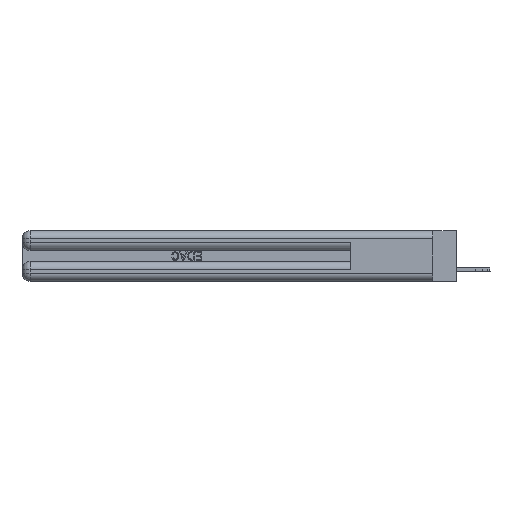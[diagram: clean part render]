
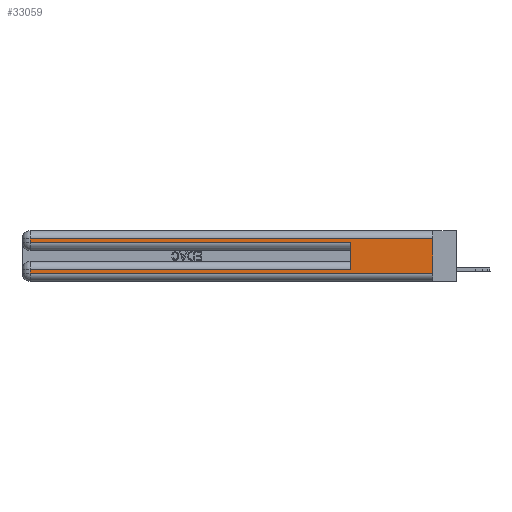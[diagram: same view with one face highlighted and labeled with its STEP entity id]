
A CAD part, left-side view. The second image highlights one B-rep face of the part: STEP entity #33059.
In plain terms, the highlighted planar face has unit normal (-1, 0, 0).
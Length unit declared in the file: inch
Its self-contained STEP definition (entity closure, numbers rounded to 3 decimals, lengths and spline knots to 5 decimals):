
#1173 = EDGE_CURVE ( 'NONE', #10407, #36564, #16976, .T. ) ;
#1502 = VECTOR ( 'NONE', #7105, 39.37008 ) ;
#1995 = ORIENTED_EDGE ( 'NONE', *, *, #1173, .T. ) ;
#2170 = DIRECTION ( 'NONE',  ( 0., -1., 0. ) ) ;
#2304 = VERTEX_POINT ( 'NONE', #34217 ) ;
#2325 = CARTESIAN_POINT ( 'NONE',  ( 0., 2.94, 0.37 ) ) ;
#3157 = DIRECTION ( 'NONE',  ( 0., 0., 1. ) ) ;
#3368 = LINE ( 'NONE', #25558, #22544 ) ;
#4999 = DIRECTION ( 'NONE',  ( 0., 1., 0. ) ) ;
#5261 = CARTESIAN_POINT ( 'NONE',  ( 0., 0., 0.085 ) ) ;
#6459 = ORIENTED_EDGE ( 'NONE', *, *, #23869, .T. ) ;
#6696 = VECTOR ( 'NONE', #2170, 39.37008 ) ;
#7105 = DIRECTION ( 'NONE',  ( 0., -1., 0. ) ) ;
#8098 = VECTOR ( 'NONE', #4999, 39.37008 ) ;
#8385 = CARTESIAN_POINT ( 'NONE',  ( 0., 2.94, 0.06 ) ) ;
#8729 = DIRECTION ( 'NONE',  ( 0., 0., -1. ) ) ;
#8767 = AXIS2_PLACEMENT_3D ( 'NONE', #23512, #29400, #26526 ) ;
#8799 = CARTESIAN_POINT ( 'NONE',  ( 0., 0., 0.06 ) ) ;
#9273 = LINE ( 'NONE', #2325, #12590 ) ;
#9824 = EDGE_CURVE ( 'NONE', #2304, #36564, #22189, .T. ) ;
#10045 = FACE_OUTER_BOUND ( 'NONE', #35761, .T. ) ;
#10250 = VECTOR ( 'NONE', #26584, 39.37008 ) ;
#10407 = VERTEX_POINT ( 'NONE', #11506 ) ;
#11506 = CARTESIAN_POINT ( 'NONE',  ( 0., 2.94, 0.285 ) ) ;
#11939 = ORIENTED_EDGE ( 'NONE', *, *, #13245, .F. ) ;
#12012 = ORIENTED_EDGE ( 'NONE', *, *, #12618, .T. ) ;
#12515 = VERTEX_POINT ( 'NONE', #8385 ) ;
#12590 = VECTOR ( 'NONE', #23504, 39.37008 ) ;
#12618 = EDGE_CURVE ( 'NONE', #2304, #25519, #18220, .T. ) ;
#13245 = EDGE_CURVE ( 'NONE', #35081, #17777, #35471, .T. ) ;
#13804 = DIRECTION ( 'NONE',  ( 0., 0., -1. ) ) ;
#13826 = ORIENTED_EDGE ( 'NONE', *, *, #18901, .T. ) ;
#15466 = CARTESIAN_POINT ( 'NONE',  ( 0., 0.6, 0.285 ) ) ;
#15667 = VECTOR ( 'NONE', #3157, 39.37008 ) ;
#15767 = CARTESIAN_POINT ( 'NONE',  ( 0., 2.94, 0.085 ) ) ;
#16155 = CARTESIAN_POINT ( 'NONE',  ( 0., 0., 0.285 ) ) ;
#16976 = LINE ( 'NONE', #16155, #1502 ) ;
#17165 = CARTESIAN_POINT ( 'NONE',  ( 0., 0., 0.31 ) ) ;
#17777 = VERTEX_POINT ( 'NONE', #8799 ) ;
#18220 = LINE ( 'NONE', #5261, #10250 ) ;
#18374 = CARTESIAN_POINT ( 'NONE',  ( 0., 2.94, 0.31 ) ) ;
#18901 = EDGE_CURVE ( 'NONE', #27694, #10407, #9273, .T. ) ;
#19485 = ORIENTED_EDGE ( 'NONE', *, *, #9824, .F. ) ;
#20130 = ORIENTED_EDGE ( 'NONE', *, *, #33897, .T. ) ;
#21968 = CARTESIAN_POINT ( 'NONE',  ( 0., 0., 0.31 ) ) ;
#22189 = LINE ( 'NONE', #35851, #15667 ) ;
#22544 = VECTOR ( 'NONE', #13804, 39.37008 ) ;
#22946 = CARTESIAN_POINT ( 'NONE',  ( 0., 0., 0.06 ) ) ;
#23504 = DIRECTION ( 'NONE',  ( 0., 0., -1. ) ) ;
#23512 = CARTESIAN_POINT ( 'NONE',  ( 0., 0., 0.37 ) ) ;
#23651 = CARTESIAN_POINT ( 'NONE',  ( 0., 0., 0.37 ) ) ;
#23869 = EDGE_CURVE ( 'NONE', #12515, #17777, #24017, .T. ) ;
#24017 = LINE ( 'NONE', #22946, #6696 ) ;
#25519 = VERTEX_POINT ( 'NONE', #15767 ) ;
#25558 = CARTESIAN_POINT ( 'NONE',  ( 0., 2.94, 0.37 ) ) ;
#26526 = DIRECTION ( 'NONE',  ( 0., 0., -1. ) ) ;
#26584 = DIRECTION ( 'NONE',  ( 0., 1., 0. ) ) ;
#27508 = VECTOR ( 'NONE', #8729, 39.37008 ) ;
#27694 = VERTEX_POINT ( 'NONE', #18374 ) ;
#29400 = DIRECTION ( 'NONE',  ( 1., 0., 0. ) ) ;
#31691 = ORIENTED_EDGE ( 'NONE', *, *, #34543, .T. ) ;
#32385 = PLANE ( 'NONE',  #8767 ) ;
#33059 = ADVANCED_FACE ( 'NONE', ( #10045 ), #32385, .F. ) ;
#33897 = EDGE_CURVE ( 'NONE', #35081, #27694, #38023, .T. ) ;
#34217 = CARTESIAN_POINT ( 'NONE',  ( 0., 0.6, 0.085 ) ) ;
#34543 = EDGE_CURVE ( 'NONE', #25519, #12515, #3368, .T. ) ;
#35081 = VERTEX_POINT ( 'NONE', #21968 ) ;
#35471 = LINE ( 'NONE', #23651, #27508 ) ;
#35761 = EDGE_LOOP ( 'NONE', ( #11939, #20130, #13826, #1995, #19485, #12012, #31691, #6459 ) ) ;
#35851 = CARTESIAN_POINT ( 'NONE',  ( 0., 0.6, 0.145 ) ) ;
#36564 = VERTEX_POINT ( 'NONE', #15466 ) ;
#38023 = LINE ( 'NONE', #17165, #8098 ) ;
